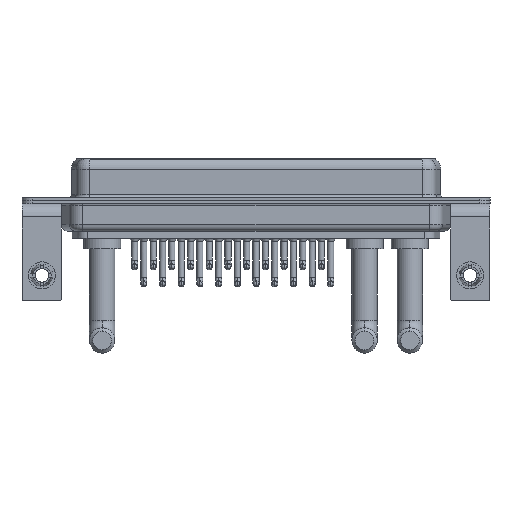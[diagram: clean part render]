
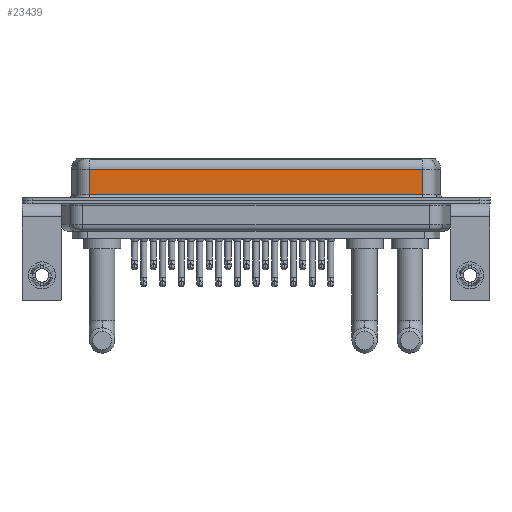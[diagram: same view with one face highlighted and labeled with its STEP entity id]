
A CAD part, front view. The second image highlights one B-rep face of the part: STEP entity #23439.
In plain terms, the highlighted planar face has unit normal (0, -1, 0).
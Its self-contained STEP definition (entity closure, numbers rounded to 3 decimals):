
#645 = CARTESIAN_POINT ( 'NONE',  ( 56.462, -3.95, 6.4 ) ) ;
#1438 = LINE ( 'NONE', #17591, #15000 ) ;
#1583 = VECTOR ( 'NONE', #4584, 1000. ) ;
#2840 = VERTEX_POINT ( 'NONE', #12078 ) ;
#2894 = FACE_OUTER_BOUND ( 'NONE', #13397, .T. ) ;
#3445 = ORIENTED_EDGE ( 'NONE', *, *, #24993, .T. ) ;
#4050 = CARTESIAN_POINT ( 'NONE',  ( 56.462, -3.95, 0.9 ) ) ;
#4584 = DIRECTION ( 'NONE',  ( 1., 0., 0. ) ) ;
#5391 = VERTEX_POINT ( 'NONE', #11203 ) ;
#8290 = LINE ( 'NONE', #4050, #1583 ) ;
#9557 = DIRECTION ( 'NONE',  ( 0., 0., -1. ) ) ;
#10105 = ORIENTED_EDGE ( 'NONE', *, *, #26038, .T. ) ;
#10261 = AXIS2_PLACEMENT_3D ( 'NONE', #645, #12834, #20906 ) ;
#11203 = CARTESIAN_POINT ( 'NONE',  ( 7.038, -3.95, 0.9 ) ) ;
#11678 = CARTESIAN_POINT ( 'NONE',  ( 56.462, -3.95, 6.4 ) ) ;
#12078 = CARTESIAN_POINT ( 'NONE',  ( 7.038, -3.95, 4.65 ) ) ;
#12708 = PLANE ( 'NONE',  #10261 ) ;
#12834 = DIRECTION ( 'NONE',  ( 0., 1., 0. ) ) ;
#12884 = VECTOR ( 'NONE', #9557, 1000. ) ;
#13397 = EDGE_LOOP ( 'NONE', ( #21342, #3445, #10105, #18316 ) ) ;
#13909 = VERTEX_POINT ( 'NONE', #24599 ) ;
#14481 = EDGE_CURVE ( 'NONE', #5391, #23238, #8290, .T. ) ;
#15000 = VECTOR ( 'NONE', #25668, 1000. ) ;
#15559 = DIRECTION ( 'NONE',  ( -1., 0., 0. ) ) ;
#17591 = CARTESIAN_POINT ( 'NONE',  ( 7.038, -3.95, 6.4 ) ) ;
#18316 = ORIENTED_EDGE ( 'NONE', *, *, #14481, .T. ) ;
#19287 = CARTESIAN_POINT ( 'NONE',  ( 56.462, -3.95, 4.65 ) ) ;
#19484 = LINE ( 'NONE', #11678, #12884 ) ;
#19547 = LINE ( 'NONE', #19287, #22593 ) ;
#20906 = DIRECTION ( 'NONE',  ( 0., 0., 1. ) ) ;
#21342 = ORIENTED_EDGE ( 'NONE', *, *, #25437, .F. ) ;
#22593 = VECTOR ( 'NONE', #15559, 1000. ) ;
#23238 = VERTEX_POINT ( 'NONE', #23734 ) ;
#23439 = ADVANCED_FACE ( 'NONE', ( #2894 ), #12708, .F. ) ;
#23734 = CARTESIAN_POINT ( 'NONE',  ( 56.462, -3.95, 0.9 ) ) ;
#24599 = CARTESIAN_POINT ( 'NONE',  ( 56.462, -3.95, 4.65 ) ) ;
#24993 = EDGE_CURVE ( 'NONE', #13909, #2840, #19547, .T. ) ;
#25437 = EDGE_CURVE ( 'NONE', #13909, #23238, #19484, .T. ) ;
#25668 = DIRECTION ( 'NONE',  ( 0., 0., -1. ) ) ;
#26038 = EDGE_CURVE ( 'NONE', #2840, #5391, #1438, .T. ) ;
